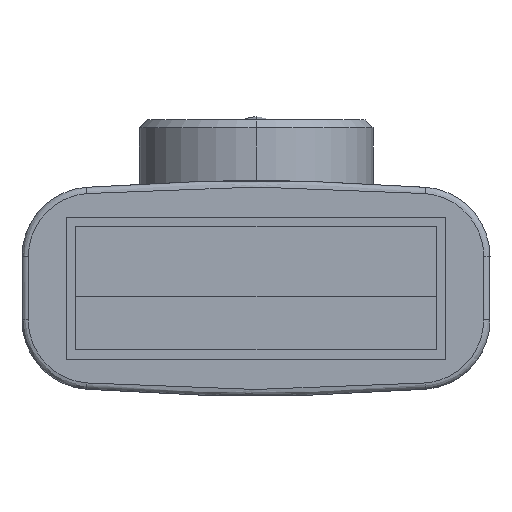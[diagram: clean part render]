
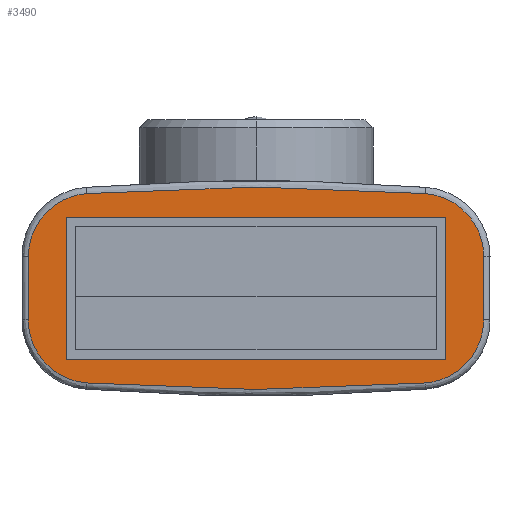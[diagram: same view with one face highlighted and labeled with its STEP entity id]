
A CAD part, front view. The second image highlights one B-rep face of the part: STEP entity #3490.
In plain terms, the highlighted planar face has unit normal (0, -1, 0).
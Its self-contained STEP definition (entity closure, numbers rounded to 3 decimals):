
#88 = EDGE_CURVE ( 'NONE', #4177, #2904, #486, .T. ) ;
#201 = VERTEX_POINT ( 'NONE', #2486 ) ;
#216 = CARTESIAN_POINT ( 'NONE',  ( 45.996, -123.781, -8.075 ) ) ;
#251 = FACE_OUTER_BOUND ( 'NONE', #3190, .T. ) ;
#403 = LINE ( 'NONE', #1327, #5212 ) ;
#486 = LINE ( 'NONE', #902, #1942 ) ;
#557 = VERTEX_POINT ( 'NONE', #1207 ) ;
#576 = CARTESIAN_POINT ( 'NONE',  ( 45.996, -123.781, -10.325 ) ) ;
#596 = CARTESIAN_POINT ( 'NONE',  ( 32.796, -123.781, -9.325 ) ) ;
#611 =( BOUNDED_CURVE ( )  B_SPLINE_CURVE ( 3, ( #1655, #1166, #2035, #3107 ),
 .UNSPECIFIED., .F., .T. ) 
 B_SPLINE_CURVE_WITH_KNOTS ( ( 4, 4 ),
 ( 0., 1. ),
 .UNSPECIFIED. ) 
 CURVE ( )  GEOMETRIC_REPRESENTATION_ITEM ( )  RATIONAL_B_SPLINE_CURVE ( ( 1., 0.822, 0.822, 1. ) ) 
 REPRESENTATION_ITEM ( '' )  );
#619 = LINE ( 'NONE', #4018, #5666 ) ;
#677 = CARTESIAN_POINT ( 'NONE',  ( 47.196, -123.781, -12.428 ) ) ;
#695 = FACE_BOUND ( 'NONE', #6248, .T. ) ;
#779 =( BOUNDED_CURVE ( )  B_SPLINE_CURVE ( 3, ( #596, #2403, #4338, #1967 ),
 .UNSPECIFIED., .F., .T. ) 
 B_SPLINE_CURVE_WITH_KNOTS ( ( 4, 4 ),
 ( 0., 1. ),
 .UNSPECIFIED. ) 
 CURVE ( )  GEOMETRIC_REPRESENTATION_ITEM ( )  RATIONAL_B_SPLINE_CURVE ( ( 1., 0.822, 0.822, 1. ) ) 
 REPRESENTATION_ITEM ( '' )  );
#827 = EDGE_CURVE ( 'NONE', #2904, #4587, #779, .T. ) ;
#858 = ORIENTED_EDGE ( 'NONE', *, *, #2883, .F. ) ;
#871 = CARTESIAN_POINT ( 'NONE',  ( 34.647, -123.781, -7.33 ) ) ;
#902 = CARTESIAN_POINT ( 'NONE',  ( 32.796, -123.781, -10.325 ) ) ;
#922 = CARTESIAN_POINT ( 'NONE',  ( 34.647, -123.781, -7.33 ) ) ;
#988 = EDGE_CURVE ( 'NONE', #3049, #201, #5436, .T. ) ;
#1098 = DIRECTION ( 'NONE',  ( 0., 0., -1. ) ) ;
#1166 = CARTESIAN_POINT ( 'NONE',  ( 46.448, -123.781, -7.415 ) ) ;
#1207 = CARTESIAN_POINT ( 'NONE',  ( 47.196, -123.781, -11.325 ) ) ;
#1327 = CARTESIAN_POINT ( 'NONE',  ( 39.996, -123.781, -8.075 ) ) ;
#1458 =( BOUNDED_CURVE ( )  B_SPLINE_CURVE ( 3, ( #4608, #677, #2201, #4102 ),
 .UNSPECIFIED., .F., .T. ) 
 B_SPLINE_CURVE_WITH_KNOTS ( ( 4, 4 ),
 ( 0., 1. ),
 .UNSPECIFIED. ) 
 CURVE ( )  GEOMETRIC_REPRESENTATION_ITEM ( )  RATIONAL_B_SPLINE_CURVE ( ( 1., 0.822, 0.822, 1. ) ) 
 REPRESENTATION_ITEM ( '' )  );
#1537 = CARTESIAN_POINT ( 'NONE',  ( 34.643, -123.781, -13.319 ) ) ;
#1567 = CARTESIAN_POINT ( 'NONE',  ( 41.785, -123.781, -7.056 ) ) ;
#1569 = CARTESIAN_POINT ( 'NONE',  ( 32.796, -123.781, -11.324 ) ) ;
#1611 = ORIENTED_EDGE ( 'NONE', *, *, #5465, .F. ) ;
#1626 = CARTESIAN_POINT ( 'NONE',  ( 45.346, -123.781, -13.32 ) ) ;
#1655 = CARTESIAN_POINT ( 'NONE',  ( 45.35, -123.781, -7.331 ) ) ;
#1677 = CARTESIAN_POINT ( 'NONE',  ( 32.796, -123.781, -11.324 ) ) ;
#1696 = ORIENTED_EDGE ( 'NONE', *, *, #988, .F. ) ;
#1758 = EDGE_CURVE ( 'NONE', #3532, #3269, #4027, .T. ) ;
#1942 = VECTOR ( 'NONE', #6251, 1000. ) ;
#1967 = CARTESIAN_POINT ( 'NONE',  ( 34.647, -123.781, -7.33 ) ) ;
#2016 = CARTESIAN_POINT ( 'NONE',  ( 33.544, -123.781, -13.235 ) ) ;
#2035 = CARTESIAN_POINT ( 'NONE',  ( 47.197, -123.781, -8.224 ) ) ;
#2088 = CARTESIAN_POINT ( 'NONE',  ( 39.996, -123.781, -12.575 ) ) ;
#2171 = VERTEX_POINT ( 'NONE', #216 ) ;
#2201 = CARTESIAN_POINT ( 'NONE',  ( 46.446, -123.781, -13.237 ) ) ;
#2322 = EDGE_CURVE ( 'NONE', #4930, #2171, #5707, .T. ) ;
#2343 = EDGE_CURVE ( 'NONE', #4587, #4694, #6227, .T. ) ;
#2359 = DIRECTION ( 'NONE',  ( 0., 0., 1. ) ) ;
#2403 = CARTESIAN_POINT ( 'NONE',  ( 32.796, -123.781, -8.221 ) ) ;
#2459 = ORIENTED_EDGE ( 'NONE', *, *, #88, .F. ) ;
#2486 = CARTESIAN_POINT ( 'NONE',  ( 33.996, -123.781, -12.575 ) ) ;
#2492 = ORIENTED_EDGE ( 'NONE', *, *, #1758, .F. ) ;
#2559 =( BOUNDED_CURVE ( )  B_SPLINE_CURVE ( 3, ( #1537, #2016, #4009, #1569 ),
 .UNSPECIFIED., .F., .T. ) 
 B_SPLINE_CURVE_WITH_KNOTS ( ( 4, 4 ),
 ( 0., 1. ),
 .UNSPECIFIED. ) 
 CURVE ( )  GEOMETRIC_REPRESENTATION_ITEM ( )  RATIONAL_B_SPLINE_CURVE ( ( 1., 0.822, 0.822, 1. ) ) 
 REPRESENTATION_ITEM ( '' )  );
#2613 = EDGE_CURVE ( 'NONE', #4694, #6157, #611, .T. ) ;
#2631 = DIRECTION ( 'NONE',  ( 0., 1., 0. ) ) ;
#2883 = EDGE_CURVE ( 'NONE', #3269, #4177, #2559, .T. ) ;
#2904 = VERTEX_POINT ( 'NONE', #5831 ) ;
#3001 = EDGE_CURVE ( 'NONE', #557, #3532, #1458, .T. ) ;
#3049 = VERTEX_POINT ( 'NONE', #3596 ) ;
#3069 = ORIENTED_EDGE ( 'NONE', *, *, #3001, .F. ) ;
#3107 = CARTESIAN_POINT ( 'NONE',  ( 47.196, -123.781, -9.326 ) ) ;
#3109 = DIRECTION ( 'NONE',  ( -1., 0., 0. ) ) ;
#3115 = CARTESIAN_POINT ( 'NONE',  ( 45.35, -123.781, -7.331 ) ) ;
#3189 = ORIENTED_EDGE ( 'NONE', *, *, #827, .F. ) ;
#3190 = EDGE_LOOP ( 'NONE', ( #4296, #5325, #3189, #2459, #858, #2492, #3069, #1611 ) ) ;
#3236 = ORIENTED_EDGE ( 'NONE', *, *, #2322, .F. ) ;
#3269 = VERTEX_POINT ( 'NONE', #5762 ) ;
#3290 = DIRECTION ( 'NONE',  ( -1., 0., 0. ) ) ;
#3490 = ADVANCED_FACE ( 'NONE', ( #251, #695 ), #5915, .F. ) ;
#3532 = VERTEX_POINT ( 'NONE', #4567 ) ;
#3545 = DIRECTION ( 'NONE',  ( 1., 0., 0. ) ) ;
#3558 = CARTESIAN_POINT ( 'NONE',  ( 34.643, -123.781, -13.319 ) ) ;
#3596 = CARTESIAN_POINT ( 'NONE',  ( 33.996, -123.781, -8.075 ) ) ;
#3598 = AXIS2_PLACEMENT_3D ( 'NONE', #4941, #2631, #3109 ) ;
#3614 = VECTOR ( 'NONE', #2359, 1000. ) ;
#3681 = CARTESIAN_POINT ( 'NONE',  ( 47.196, -123.781, -9.326 ) ) ;
#3833 = CARTESIAN_POINT ( 'NONE',  ( 45.996, -123.781, -12.575 ) ) ;
#3908 = CARTESIAN_POINT ( 'NONE',  ( 45.35, -123.781, -7.331 ) ) ;
#3924 = EDGE_CURVE ( 'NONE', #201, #4930, #4082, .T. ) ;
#4009 = CARTESIAN_POINT ( 'NONE',  ( 32.795, -123.781, -12.426 ) ) ;
#4018 = CARTESIAN_POINT ( 'NONE',  ( 47.196, -123.781, -10.325 ) ) ;
#4027 =( BOUNDED_CURVE ( )  B_SPLINE_CURVE ( 3, ( #1626, #4943, #4066, #3558 ),
 .UNSPECIFIED., .F., .T. ) 
 B_SPLINE_CURVE_WITH_KNOTS ( ( 4, 4 ),
 ( 0., 1. ),
 .UNSPECIFIED. ) 
 CURVE ( )  GEOMETRIC_REPRESENTATION_ITEM ( )  RATIONAL_B_SPLINE_CURVE ( ( 1., 0.998, 0.998, 1. ) ) 
 REPRESENTATION_ITEM ( '' )  );
#4066 = CARTESIAN_POINT ( 'NONE',  ( 38.207, -123.781, -13.594 ) ) ;
#4082 = LINE ( 'NONE', #2088, #4812 ) ;
#4102 = CARTESIAN_POINT ( 'NONE',  ( 45.346, -123.781, -13.32 ) ) ;
#4177 = VERTEX_POINT ( 'NONE', #1677 ) ;
#4181 = ORIENTED_EDGE ( 'NONE', *, *, #4305, .F. ) ;
#4296 = ORIENTED_EDGE ( 'NONE', *, *, #2613, .F. ) ;
#4305 = EDGE_CURVE ( 'NONE', #2171, #3049, #403, .T. ) ;
#4338 = CARTESIAN_POINT ( 'NONE',  ( 33.547, -123.781, -7.413 ) ) ;
#4415 = CARTESIAN_POINT ( 'NONE',  ( 38.211, -123.781, -7.056 ) ) ;
#4467 = CARTESIAN_POINT ( 'NONE',  ( 33.996, -123.781, -10.325 ) ) ;
#4567 = CARTESIAN_POINT ( 'NONE',  ( 45.346, -123.781, -13.32 ) ) ;
#4587 = VERTEX_POINT ( 'NONE', #922 ) ;
#4608 = CARTESIAN_POINT ( 'NONE',  ( 47.196, -123.781, -11.325 ) ) ;
#4694 = VERTEX_POINT ( 'NONE', #3115 ) ;
#4810 = VECTOR ( 'NONE', #1098, 1000. ) ;
#4812 = VECTOR ( 'NONE', #3545, 1000. ) ;
#4930 = VERTEX_POINT ( 'NONE', #3833 ) ;
#4941 = CARTESIAN_POINT ( 'NONE',  ( 39.996, -123.781, -10.325 ) ) ;
#4943 = CARTESIAN_POINT ( 'NONE',  ( 41.782, -123.781, -13.594 ) ) ;
#5212 = VECTOR ( 'NONE', #3290, 1000. ) ;
#5325 = ORIENTED_EDGE ( 'NONE', *, *, #2343, .F. ) ;
#5436 = LINE ( 'NONE', #4467, #4810 ) ;
#5465 = EDGE_CURVE ( 'NONE', #6157, #557, #619, .T. ) ;
#5666 = VECTOR ( 'NONE', #5872, 1000. ) ;
#5707 = LINE ( 'NONE', #576, #3614 ) ;
#5717 = ORIENTED_EDGE ( 'NONE', *, *, #3924, .F. ) ;
#5762 = CARTESIAN_POINT ( 'NONE',  ( 34.643, -123.781, -13.319 ) ) ;
#5831 = CARTESIAN_POINT ( 'NONE',  ( 32.796, -123.781, -9.325 ) ) ;
#5872 = DIRECTION ( 'NONE',  ( 0., 0., -1. ) ) ;
#5915 = PLANE ( 'NONE',  #3598 ) ;
#6157 = VERTEX_POINT ( 'NONE', #3681 ) ;
#6227 =( BOUNDED_CURVE ( )  B_SPLINE_CURVE ( 3, ( #871, #4415, #1567, #3908 ),
 .UNSPECIFIED., .F., .T. ) 
 B_SPLINE_CURVE_WITH_KNOTS ( ( 4, 4 ),
 ( 0., 1. ),
 .UNSPECIFIED. ) 
 CURVE ( )  GEOMETRIC_REPRESENTATION_ITEM ( )  RATIONAL_B_SPLINE_CURVE ( ( 1., 0.998, 0.998, 1. ) ) 
 REPRESENTATION_ITEM ( '' )  );
#6248 = EDGE_LOOP ( 'NONE', ( #3236, #5717, #1696, #4181 ) ) ;
#6251 = DIRECTION ( 'NONE',  ( 0., 0., 1. ) ) ;
